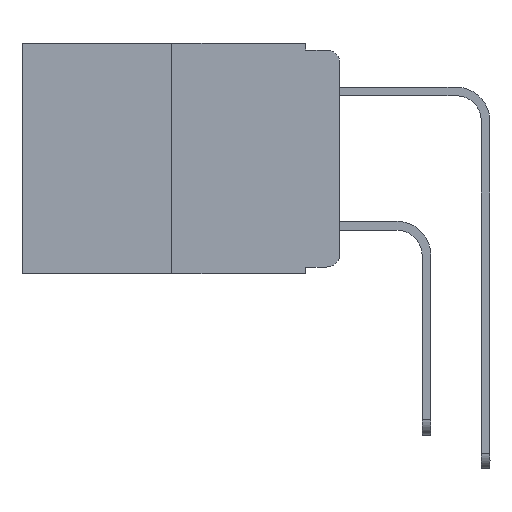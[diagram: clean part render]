
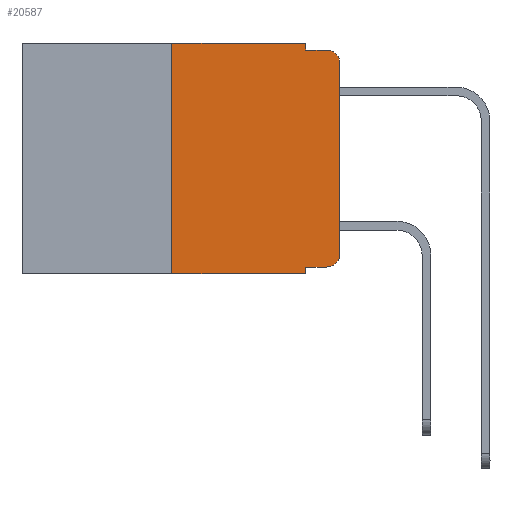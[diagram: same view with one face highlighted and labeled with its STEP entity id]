
A CAD part, left-side view. The second image highlights one B-rep face of the part: STEP entity #20587.
In plain terms, the highlighted planar face has unit normal (-1, 0, 0).
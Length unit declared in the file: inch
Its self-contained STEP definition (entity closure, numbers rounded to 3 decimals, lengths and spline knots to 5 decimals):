
#240 = EDGE_CURVE ( 'NONE', #2650, #9362, #18572, .T. ) ;
#508 = CARTESIAN_POINT ( 'NONE',  ( 0., 0.051, 0. ) ) ;
#1633 = LINE ( 'NONE', #6897, #12898 ) ;
#1896 = DIRECTION ( 'NONE',  ( 0., -1., 0. ) ) ;
#1918 = EDGE_CURVE ( 'NONE', #15437, #6498, #2326, .T. ) ;
#2154 = CARTESIAN_POINT ( 'NONE',  ( 0., 0.051, -0.01 ) ) ;
#2326 = LINE ( 'NONE', #9091, #12499 ) ;
#2432 = VECTOR ( 'NONE', #8824, 39.37008 ) ;
#2600 = VECTOR ( 'NONE', #5414, 39.37008 ) ;
#2650 = VERTEX_POINT ( 'NONE', #7186 ) ;
#2696 = EDGE_CURVE ( 'NONE', #9456, #5252, #7399, .T. ) ;
#3091 = CARTESIAN_POINT ( 'NONE',  ( 0., 0.051, -0.333 ) ) ;
#3299 = CARTESIAN_POINT ( 'NONE',  ( 0., 0.051, 0. ) ) ;
#3504 = DIRECTION ( 'NONE',  ( 1., 0., 0. ) ) ;
#4345 = ORIENTED_EDGE ( 'NONE', *, *, #1918, .F. ) ;
#4684 = DIRECTION ( 'NONE',  ( -1., 0., 0. ) ) ;
#4727 = VERTEX_POINT ( 'NONE', #3091 ) ;
#4737 = AXIS2_PLACEMENT_3D ( 'NONE', #6305, #16283, #12839 ) ;
#4787 = CARTESIAN_POINT ( 'NONE',  ( 0., 0.25, 0. ) ) ;
#4917 = LINE ( 'NONE', #18007, #17954 ) ;
#5241 = LINE ( 'NONE', #508, #7481 ) ;
#5252 = VERTEX_POINT ( 'NONE', #6710 ) ;
#5414 = DIRECTION ( 'NONE',  ( 0., 0., -1. ) ) ;
#5614 = CARTESIAN_POINT ( 'NONE',  ( 0., 0.25, -0.343 ) ) ;
#5726 = EDGE_CURVE ( 'NONE', #4727, #8247, #1633, .T. ) ;
#6305 = CARTESIAN_POINT ( 'NONE',  ( 0., 0.02, -0.313 ) ) ;
#6498 = VERTEX_POINT ( 'NONE', #4787 ) ;
#6710 = CARTESIAN_POINT ( 'NONE',  ( 0., 0., -0.03 ) ) ;
#6897 = CARTESIAN_POINT ( 'NONE',  ( 0., 0.051, -0.333 ) ) ;
#7062 = DIRECTION ( 'NONE',  ( 0., 0., -1. ) ) ;
#7186 = CARTESIAN_POINT ( 'NONE',  ( 0., 0.051, -0.01 ) ) ;
#7399 = LINE ( 'NONE', #7716, #15686 ) ;
#7481 = VECTOR ( 'NONE', #7062, 39.37008 ) ;
#7654 = ORIENTED_EDGE ( 'NONE', *, *, #16641, .T. ) ;
#7716 = CARTESIAN_POINT ( 'NONE',  ( 0., 0., 0. ) ) ;
#7898 = AXIS2_PLACEMENT_3D ( 'NONE', #19375, #4684, #14558 ) ;
#8194 = DIRECTION ( 'NONE',  ( 0., -1., 0. ) ) ;
#8247 = VERTEX_POINT ( 'NONE', #21175 ) ;
#8824 = DIRECTION ( 'NONE',  ( 0., -1., 0. ) ) ;
#8865 = CIRCLE ( 'NONE', #4737, 0.02 ) ;
#8878 = DIRECTION ( 'NONE',  ( 0., 0., -1. ) ) ;
#9003 = CARTESIAN_POINT ( 'NONE',  ( 0., 0.051, -0.343 ) ) ;
#9024 = ORIENTED_EDGE ( 'NONE', *, *, #12395, .F. ) ;
#9091 = CARTESIAN_POINT ( 'NONE',  ( 0., 0.25, 0. ) ) ;
#9114 = DIRECTION ( 'NONE',  ( 0., 0., 1. ) ) ;
#9362 = VERTEX_POINT ( 'NONE', #18128 ) ;
#9456 = VERTEX_POINT ( 'NONE', #16954 ) ;
#9764 = EDGE_CURVE ( 'NONE', #4727, #11306, #19995, .T. ) ;
#9871 = VECTOR ( 'NONE', #1896, 39.37008 ) ;
#10073 = LINE ( 'NONE', #16617, #9871 ) ;
#11306 = VERTEX_POINT ( 'NONE', #9003 ) ;
#11436 = EDGE_LOOP ( 'NONE', ( #12634, #7654, #14073, #9024, #15723, #4345, #20830, #18766, #15501, #17122 ) ) ;
#11505 = AXIS2_PLACEMENT_3D ( 'NONE', #15418, #3504, #8878 ) ;
#12215 = CARTESIAN_POINT ( 'NONE',  ( 0., 0.051, 0. ) ) ;
#12395 = EDGE_CURVE ( 'NONE', #12593, #2650, #5241, .T. ) ;
#12463 = EDGE_CURVE ( 'NONE', #6498, #12593, #10073, .T. ) ;
#12499 = VECTOR ( 'NONE', #15429, 39.37008 ) ;
#12593 = VERTEX_POINT ( 'NONE', #12215 ) ;
#12634 = ORIENTED_EDGE ( 'NONE', *, *, #2696, .T. ) ;
#12792 = EDGE_CURVE ( 'NONE', #8247, #9456, #8865, .T. ) ;
#12839 = DIRECTION ( 'NONE',  ( 0., 0., -1. ) ) ;
#12898 = VECTOR ( 'NONE', #8194, 39.37008 ) ;
#14073 = ORIENTED_EDGE ( 'NONE', *, *, #240, .F. ) ;
#14558 = DIRECTION ( 'NONE',  ( 0., 0., -1. ) ) ;
#14796 = DIRECTION ( 'NONE',  ( 0., -1., 0. ) ) ;
#15418 = CARTESIAN_POINT ( 'NONE',  ( 0., 0.473, 0. ) ) ;
#15429 = DIRECTION ( 'NONE',  ( 0., 0., 1. ) ) ;
#15437 = VERTEX_POINT ( 'NONE', #5614 ) ;
#15501 = ORIENTED_EDGE ( 'NONE', *, *, #5726, .T. ) ;
#15686 = VECTOR ( 'NONE', #9114, 39.37008 ) ;
#15723 = ORIENTED_EDGE ( 'NONE', *, *, #12463, .F. ) ;
#16283 = DIRECTION ( 'NONE',  ( -1., 0., 0. ) ) ;
#16617 = CARTESIAN_POINT ( 'NONE',  ( 0., 0.473, 0. ) ) ;
#16641 = EDGE_CURVE ( 'NONE', #5252, #9362, #18170, .T. ) ;
#16918 = PLANE ( 'NONE',  #11505 ) ;
#16954 = CARTESIAN_POINT ( 'NONE',  ( 0., 0., -0.313 ) ) ;
#17122 = ORIENTED_EDGE ( 'NONE', *, *, #12792, .T. ) ;
#17954 = VECTOR ( 'NONE', #14796, 39.37008 ) ;
#18007 = CARTESIAN_POINT ( 'NONE',  ( 0., 0.473, -0.343 ) ) ;
#18128 = CARTESIAN_POINT ( 'NONE',  ( 0., 0.02, -0.01 ) ) ;
#18170 = CIRCLE ( 'NONE', #7898, 0.02 ) ;
#18572 = LINE ( 'NONE', #2154, #2432 ) ;
#18766 = ORIENTED_EDGE ( 'NONE', *, *, #9764, .F. ) ;
#19375 = CARTESIAN_POINT ( 'NONE',  ( 0., 0.02, -0.03 ) ) ;
#19995 = LINE ( 'NONE', #3299, #2600 ) ;
#20121 = EDGE_CURVE ( 'NONE', #15437, #11306, #4917, .T. ) ;
#20224 = FACE_OUTER_BOUND ( 'NONE', #11436, .T. ) ;
#20587 = ADVANCED_FACE ( 'NONE', ( #20224 ), #16918, .F. ) ;
#20830 = ORIENTED_EDGE ( 'NONE', *, *, #20121, .T. ) ;
#21175 = CARTESIAN_POINT ( 'NONE',  ( 0., 0.02, -0.333 ) ) ;
